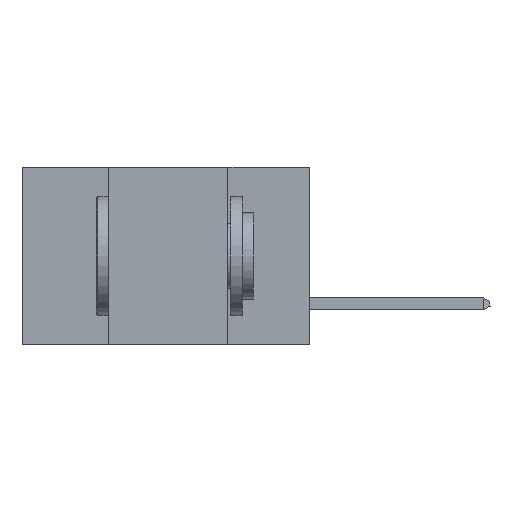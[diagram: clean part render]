
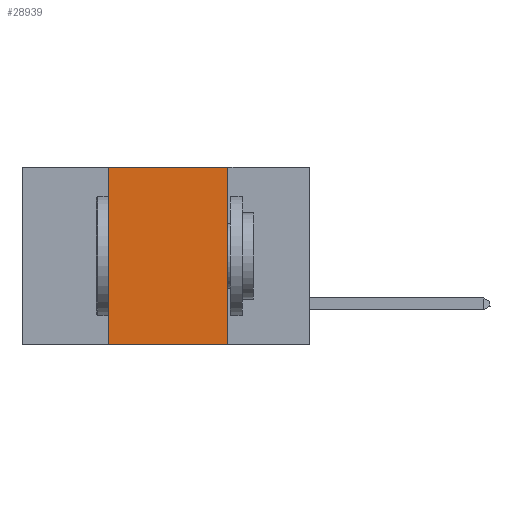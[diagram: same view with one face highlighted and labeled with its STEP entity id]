
A CAD part, left-side view. The second image highlights one B-rep face of the part: STEP entity #28939.
In plain terms, the highlighted planar face has unit normal (-1, 0, 0).
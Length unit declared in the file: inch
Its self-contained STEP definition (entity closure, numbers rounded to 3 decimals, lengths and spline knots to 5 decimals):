
#428 = DIRECTION ( 'NONE',  ( 0., -1., 0. ) ) ;
#949 = VERTEX_POINT ( 'NONE', #14198 ) ;
#1809 = LINE ( 'NONE', #17595, #22575 ) ;
#2050 = DIRECTION ( 'NONE',  ( 1., 0., 0. ) ) ;
#2792 = LINE ( 'NONE', #7349, #12676 ) ;
#2934 = VERTEX_POINT ( 'NONE', #35908 ) ;
#3073 = DIRECTION ( 'NONE',  ( 0., 0., 1. ) ) ;
#4110 = AXIS2_PLACEMENT_3D ( 'NONE', #33595, #2050, #16287 ) ;
#6226 = VERTEX_POINT ( 'NONE', #12792 ) ;
#6631 = EDGE_CURVE ( 'NONE', #2934, #26907, #11381, .T. ) ;
#7190 = ORIENTED_EDGE ( 'NONE', *, *, #29362, .F. ) ;
#7349 = CARTESIAN_POINT ( 'NONE',  ( 0., 0.17, 0. ) ) ;
#8736 = VECTOR ( 'NONE', #13573, 39.37008 ) ;
#10073 = DIRECTION ( 'NONE',  ( 0., 0., -1. ) ) ;
#10387 = ORIENTED_EDGE ( 'NONE', *, *, #24052, .T. ) ;
#10581 = CARTESIAN_POINT ( 'NONE',  ( 0., 0.42, 0. ) ) ;
#10643 = CARTESIAN_POINT ( 'NONE',  ( 0., 0.6, -0.37 ) ) ;
#11381 = LINE ( 'NONE', #22970, #35757 ) ;
#12676 = VECTOR ( 'NONE', #10073, 39.37008 ) ;
#12792 = CARTESIAN_POINT ( 'NONE',  ( 0., 0.17, -0.37 ) ) ;
#13573 = DIRECTION ( 'NONE',  ( 0., -1., 0. ) ) ;
#14198 = CARTESIAN_POINT ( 'NONE',  ( 0., 0.17, 0. ) ) ;
#15130 = FACE_OUTER_BOUND ( 'NONE', #19915, .T. ) ;
#16287 = DIRECTION ( 'NONE',  ( 0., 0., -1. ) ) ;
#17595 = CARTESIAN_POINT ( 'NONE',  ( 0., 0.6, 0. ) ) ;
#19915 = EDGE_LOOP ( 'NONE', ( #7190, #33993, #28937, #10387 ) ) ;
#20911 = LINE ( 'NONE', #10643, #8736 ) ;
#22575 = VECTOR ( 'NONE', #428, 39.37008 ) ;
#22970 = CARTESIAN_POINT ( 'NONE',  ( 0., 0.42, 0. ) ) ;
#24052 = EDGE_CURVE ( 'NONE', #2934, #6226, #20911, .T. ) ;
#25821 = EDGE_CURVE ( 'NONE', #26907, #949, #1809, .T. ) ;
#26907 = VERTEX_POINT ( 'NONE', #10581 ) ;
#28937 = ORIENTED_EDGE ( 'NONE', *, *, #6631, .F. ) ;
#28939 = ADVANCED_FACE ( 'NONE', ( #15130 ), #36609, .F. ) ;
#29362 = EDGE_CURVE ( 'NONE', #949, #6226, #2792, .T. ) ;
#33595 = CARTESIAN_POINT ( 'NONE',  ( 0., 0.6, 0. ) ) ;
#33993 = ORIENTED_EDGE ( 'NONE', *, *, #25821, .F. ) ;
#35757 = VECTOR ( 'NONE', #3073, 39.37008 ) ;
#35908 = CARTESIAN_POINT ( 'NONE',  ( 0., 0.42, -0.37 ) ) ;
#36609 = PLANE ( 'NONE',  #4110 ) ;
